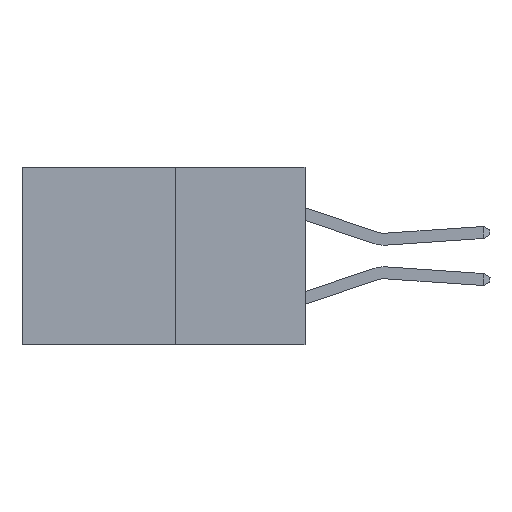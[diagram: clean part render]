
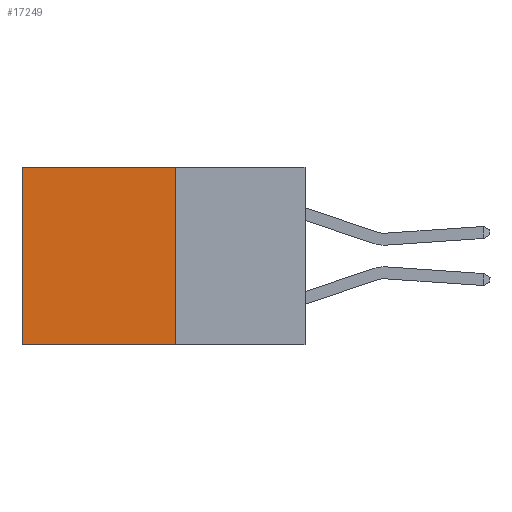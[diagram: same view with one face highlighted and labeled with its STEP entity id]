
A CAD part, left-side view. The second image highlights one B-rep face of the part: STEP entity #17249.
In plain terms, the highlighted planar face has unit normal (-1, 0, 0).
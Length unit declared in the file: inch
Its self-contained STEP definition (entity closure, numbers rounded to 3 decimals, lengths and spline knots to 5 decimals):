
#354 = DIRECTION ( 'NONE',  ( 1., 0., 0. ) ) ;
#607 = ORIENTED_EDGE ( 'NONE', *, *, #7812, .F. ) ;
#1106 = CARTESIAN_POINT ( 'NONE',  ( 0.277, 0.27, -0.37 ) ) ;
#2546 = VERTEX_POINT ( 'NONE', #17932 ) ;
#2746 = ORIENTED_EDGE ( 'NONE', *, *, #33549, .T. ) ;
#3787 = VERTEX_POINT ( 'NONE', #1106 ) ;
#3914 = VERTEX_POINT ( 'NONE', #33662 ) ;
#4577 = LINE ( 'NONE', #17238, #11051 ) ;
#7287 = LINE ( 'NONE', #13792, #21010 ) ;
#7812 = EDGE_CURVE ( 'NONE', #2546, #3787, #29381, .T. ) ;
#9788 = VECTOR ( 'NONE', #33135, 39.37008 ) ;
#11051 = VECTOR ( 'NONE', #33478, 39.37008 ) ;
#12465 = VERTEX_POINT ( 'NONE', #21993 ) ;
#13792 = CARTESIAN_POINT ( 'NONE',  ( 0.277, 0.27, -0.37 ) ) ;
#14137 = CARTESIAN_POINT ( 'NONE',  ( 0.277, 0.27, 0. ) ) ;
#14683 = EDGE_LOOP ( 'NONE', ( #2746, #19988, #607, #25102 ) ) ;
#15708 = EDGE_CURVE ( 'NONE', #3787, #3914, #7287, .T. ) ;
#16569 = DIRECTION ( 'NONE',  ( 0., 1., 0. ) ) ;
#16867 = CARTESIAN_POINT ( 'NONE',  ( 0.277, 0.27, -0.37 ) ) ;
#17238 = CARTESIAN_POINT ( 'NONE',  ( 0.277, 0.59, -0.37 ) ) ;
#17249 = ADVANCED_FACE ( 'NONE', ( #20295 ), #33105, .F. ) ;
#17390 = AXIS2_PLACEMENT_3D ( 'NONE', #16867, #354, #19628 ) ;
#17932 = CARTESIAN_POINT ( 'NONE',  ( 0.277, 0.27, 0. ) ) ;
#19628 = DIRECTION ( 'NONE',  ( 0., 0., -1. ) ) ;
#19988 = ORIENTED_EDGE ( 'NONE', *, *, #15708, .F. ) ;
#20295 = FACE_OUTER_BOUND ( 'NONE', #14683, .T. ) ;
#21010 = VECTOR ( 'NONE', #16569, 39.37008 ) ;
#21993 = CARTESIAN_POINT ( 'NONE',  ( 0.277, 0.59, 0. ) ) ;
#25102 = ORIENTED_EDGE ( 'NONE', *, *, #25296, .T. ) ;
#25296 = EDGE_CURVE ( 'NONE', #2546, #12465, #31517, .T. ) ;
#28510 = VECTOR ( 'NONE', #30562, 39.37008 ) ;
#29381 = LINE ( 'NONE', #30840, #28510 ) ;
#30562 = DIRECTION ( 'NONE',  ( 0., 0., -1. ) ) ;
#30840 = CARTESIAN_POINT ( 'NONE',  ( 0.277, 0.27, -0.37 ) ) ;
#31517 = LINE ( 'NONE', #14137, #9788 ) ;
#33105 = PLANE ( 'NONE',  #17390 ) ;
#33135 = DIRECTION ( 'NONE',  ( 0., 1., 0. ) ) ;
#33478 = DIRECTION ( 'NONE',  ( 0., 0., -1. ) ) ;
#33549 = EDGE_CURVE ( 'NONE', #12465, #3914, #4577, .T. ) ;
#33662 = CARTESIAN_POINT ( 'NONE',  ( 0.277, 0.59, -0.37 ) ) ;
